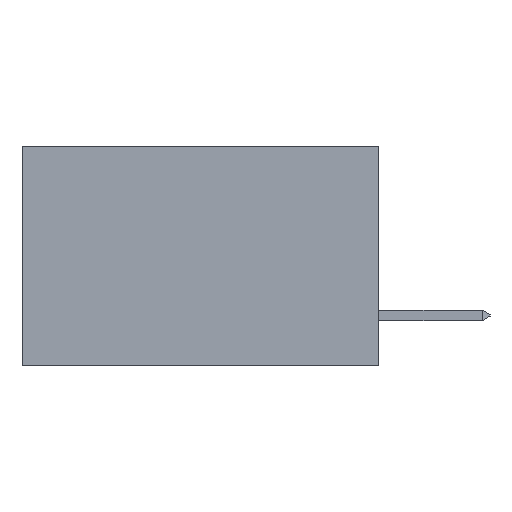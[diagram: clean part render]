
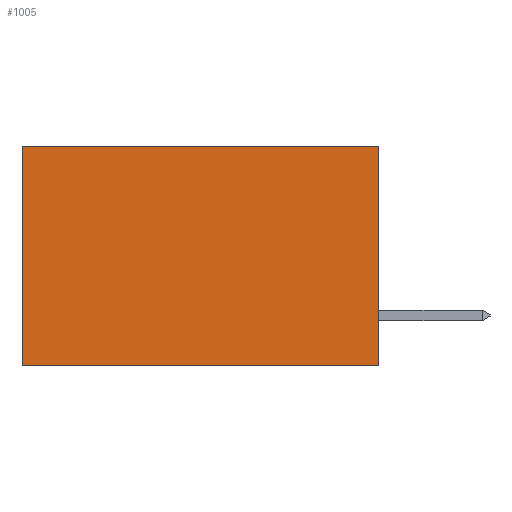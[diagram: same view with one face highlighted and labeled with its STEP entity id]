
A CAD part, left-side view. The second image highlights one B-rep face of the part: STEP entity #1005.
In plain terms, the highlighted planar face has unit normal (-1, 0, 0).
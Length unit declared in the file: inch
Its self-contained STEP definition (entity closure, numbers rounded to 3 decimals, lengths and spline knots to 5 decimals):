
#683 = ORIENTED_EDGE ( 'NONE', *, *, #4790, .T. ) ;
#1005 = ADVANCED_FACE ( 'NONE', ( #9624 ), #10504, .F. ) ;
#1134 = LINE ( 'NONE', #2953, #8599 ) ;
#1978 = DIRECTION ( 'NONE',  ( 0., 0., -1. ) ) ;
#2953 = CARTESIAN_POINT ( 'NONE',  ( 0.2615, 0., 0. ) ) ;
#3989 = CARTESIAN_POINT ( 'NONE',  ( 0.2615, 0.6, 0. ) ) ;
#4472 = DIRECTION ( 'NONE',  ( 0., 1., 0. ) ) ;
#4790 = EDGE_CURVE ( 'NONE', #17301, #4911, #5728, .T. ) ;
#4911 = VERTEX_POINT ( 'NONE', #9337 ) ;
#5063 = DIRECTION ( 'NONE',  ( 0., 0., -1. ) ) ;
#5728 = LINE ( 'NONE', #13986, #13408 ) ;
#5839 = EDGE_CURVE ( 'NONE', #12727, #4911, #12266, .T. ) ;
#6464 = VECTOR ( 'NONE', #1978, 39.37008 ) ;
#7060 = DIRECTION ( 'NONE',  ( 1., 0., 0. ) ) ;
#7095 = EDGE_LOOP ( 'NONE', ( #683, #10676, #17359, #11599 ) ) ;
#8036 = VECTOR ( 'NONE', #10874, 39.37008 ) ;
#8366 = CARTESIAN_POINT ( 'NONE',  ( 0.2615, 0., -0.37 ) ) ;
#8599 = VECTOR ( 'NONE', #4472, 39.37008 ) ;
#9337 = CARTESIAN_POINT ( 'NONE',  ( 0.2615, 0.6, -0.37 ) ) ;
#9428 = CARTESIAN_POINT ( 'NONE',  ( 0.2615, 0., -0.37 ) ) ;
#9624 = FACE_OUTER_BOUND ( 'NONE', #7095, .T. ) ;
#10504 = PLANE ( 'NONE',  #11206 ) ;
#10676 = ORIENTED_EDGE ( 'NONE', *, *, #5839, .F. ) ;
#10874 = DIRECTION ( 'NONE',  ( 0., 1., 0. ) ) ;
#10912 = CARTESIAN_POINT ( 'NONE',  ( 0.2615, 0., -0.37 ) ) ;
#11206 = AXIS2_PLACEMENT_3D ( 'NONE', #8366, #7060, #5063 ) ;
#11599 = ORIENTED_EDGE ( 'NONE', *, *, #11918, .T. ) ;
#11918 = EDGE_CURVE ( 'NONE', #15947, #17301, #1134, .T. ) ;
#12266 = LINE ( 'NONE', #10912, #8036 ) ;
#12727 = VERTEX_POINT ( 'NONE', #15560 ) ;
#13408 = VECTOR ( 'NONE', #13961, 39.37008 ) ;
#13961 = DIRECTION ( 'NONE',  ( 0., 0., -1. ) ) ;
#13986 = CARTESIAN_POINT ( 'NONE',  ( 0.2615, 0.6, -0.37 ) ) ;
#15560 = CARTESIAN_POINT ( 'NONE',  ( 0.2615, 0., -0.37 ) ) ;
#15947 = VERTEX_POINT ( 'NONE', #17064 ) ;
#17064 = CARTESIAN_POINT ( 'NONE',  ( 0.2615, 0., 0. ) ) ;
#17301 = VERTEX_POINT ( 'NONE', #3989 ) ;
#17359 = ORIENTED_EDGE ( 'NONE', *, *, #17728, .F. ) ;
#17728 = EDGE_CURVE ( 'NONE', #15947, #12727, #17872, .T. ) ;
#17872 = LINE ( 'NONE', #9428, #6464 ) ;
